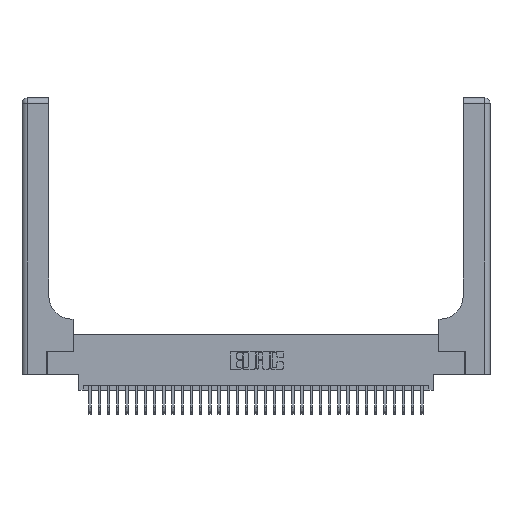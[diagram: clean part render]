
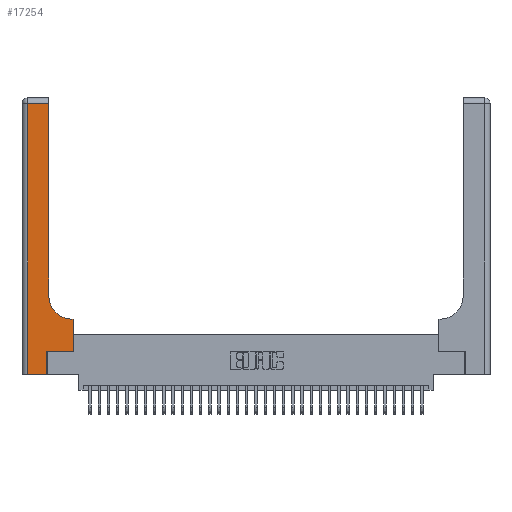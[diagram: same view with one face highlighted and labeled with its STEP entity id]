
A CAD part, top view. The second image highlights one B-rep face of the part: STEP entity #17254.
In plain terms, the highlighted planar face has unit normal (0, 0, 1).
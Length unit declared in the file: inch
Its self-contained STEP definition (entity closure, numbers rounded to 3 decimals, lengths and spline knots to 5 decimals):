
#334 = AXIS2_PLACEMENT_3D ( 'NONE', #34605, #17722, #707 ) ;
#538 = CARTESIAN_POINT ( 'NONE',  ( 0.2915, 0.85, 0.37 ) ) ;
#707 = DIRECTION ( 'NONE',  ( -1., 0., 0. ) ) ;
#1092 = VERTEX_POINT ( 'NONE', #1287 ) ;
#1287 = CARTESIAN_POINT ( 'NONE',  ( 0.269, 0.25, 0.37 ) ) ;
#1878 = EDGE_CURVE ( 'NONE', #11000, #27394, #16429, .T. ) ;
#2353 = EDGE_LOOP ( 'NONE', ( #31193, #34270, #35173, #10606, #19330, #17640, #6904, #22198, #26988 ) ) ;
#4178 = DIRECTION ( 'NONE',  ( 0., 1., 0. ) ) ;
#4311 = EDGE_CURVE ( 'NONE', #13612, #11000, #26911, .T. ) ;
#4938 = LINE ( 'NONE', #35221, #19146 ) ;
#4997 = EDGE_CURVE ( 'NONE', #1092, #9421, #5575, .T. ) ;
#5121 = VERTEX_POINT ( 'NONE', #24001 ) ;
#5575 = LINE ( 'NONE', #29184, #13089 ) ;
#6449 = LINE ( 'NONE', #24709, #34694 ) ;
#6904 = ORIENTED_EDGE ( 'NONE', *, *, #28859, .T. ) ;
#7511 = LINE ( 'NONE', #23362, #35757 ) ;
#8541 = CARTESIAN_POINT ( 'NONE',  ( 0.2915, 2.94, 0.37 ) ) ;
#8618 = EDGE_CURVE ( 'NONE', #27394, #20271, #6449, .T. ) ;
#9202 = PLANE ( 'NONE',  #334 ) ;
#9421 = VERTEX_POINT ( 'NONE', #15098 ) ;
#10004 = AXIS2_PLACEMENT_3D ( 'NONE', #10702, #30483, #13531 ) ;
#10589 = DIRECTION ( 'NONE',  ( 0., 1., 0. ) ) ;
#10606 = ORIENTED_EDGE ( 'NONE', *, *, #31074, .T. ) ;
#10702 = CARTESIAN_POINT ( 'NONE',  ( 0.5415, 0.85, 0.37 ) ) ;
#11000 = VERTEX_POINT ( 'NONE', #36220 ) ;
#12005 = DIRECTION ( 'NONE',  ( -1., 0., 0. ) ) ;
#12429 = CARTESIAN_POINT ( 'NONE',  ( 0.06, 2.94, 0.37 ) ) ;
#13089 = VECTOR ( 'NONE', #15062, 39.37008 ) ;
#13531 = DIRECTION ( 'NONE',  ( 1., 0., 0. ) ) ;
#13612 = VERTEX_POINT ( 'NONE', #30151 ) ;
#13981 = DIRECTION ( 'NONE',  ( -1., 0., 0. ) ) ;
#14082 = VECTOR ( 'NONE', #15932, 39.37008 ) ;
#14226 = FACE_OUTER_BOUND ( 'NONE', #2353, .T. ) ;
#14783 = DIRECTION ( 'NONE',  ( 0., -1., 0. ) ) ;
#14954 = LINE ( 'NONE', #35663, #14082 ) ;
#15062 = DIRECTION ( 'NONE',  ( 1., 0., 0. ) ) ;
#15098 = CARTESIAN_POINT ( 'NONE',  ( 0.5585, 0.25, 0.37 ) ) ;
#15932 = DIRECTION ( 'NONE',  ( 1., 0., 0. ) ) ;
#16429 = CIRCLE ( 'NONE', #10004, 0.25 ) ;
#17254 = ADVANCED_FACE ( 'NONE', ( #14226 ), #9202, .F. ) ;
#17640 = ORIENTED_EDGE ( 'NONE', *, *, #4997, .T. ) ;
#17712 = CARTESIAN_POINT ( 'NONE',  ( 0.2915, 0.6, 0.37 ) ) ;
#17722 = DIRECTION ( 'NONE',  ( 0., 0., -1. ) ) ;
#19146 = VECTOR ( 'NONE', #4178, 39.37008 ) ;
#19330 = ORIENTED_EDGE ( 'NONE', *, *, #27661, .T. ) ;
#20271 = VERTEX_POINT ( 'NONE', #8541 ) ;
#20566 = LINE ( 'NONE', #30052, #21463 ) ;
#21463 = VECTOR ( 'NONE', #32751, 39.37008 ) ;
#22198 = ORIENTED_EDGE ( 'NONE', *, *, #4311, .T. ) ;
#23362 = CARTESIAN_POINT ( 'NONE',  ( 0.06, 3., 0.37 ) ) ;
#24001 = CARTESIAN_POINT ( 'NONE',  ( 0.269, 0., 0.37 ) ) ;
#24709 = CARTESIAN_POINT ( 'NONE',  ( 0.2915, 3., 0.37 ) ) ;
#25024 = CARTESIAN_POINT ( 'NONE',  ( 0., 2.94, 0.37 ) ) ;
#26911 = LINE ( 'NONE', #17712, #33496 ) ;
#26988 = ORIENTED_EDGE ( 'NONE', *, *, #1878, .T. ) ;
#27394 = VERTEX_POINT ( 'NONE', #538 ) ;
#27661 = EDGE_CURVE ( 'NONE', #5121, #1092, #20566, .T. ) ;
#27914 = CARTESIAN_POINT ( 'NONE',  ( 0.06, 0., 0.37 ) ) ;
#27997 = LINE ( 'NONE', #25024, #35433 ) ;
#28859 = EDGE_CURVE ( 'NONE', #9421, #13612, #4938, .T. ) ;
#29081 = EDGE_CURVE ( 'NONE', #20271, #34041, #27997, .T. ) ;
#29184 = CARTESIAN_POINT ( 'NONE',  ( 0.269, 0.25, 0.37 ) ) ;
#30052 = CARTESIAN_POINT ( 'NONE',  ( 0.269, 0., 0.37 ) ) ;
#30151 = CARTESIAN_POINT ( 'NONE',  ( 0.5585, 0.6, 0.37 ) ) ;
#30483 = DIRECTION ( 'NONE',  ( 0., 0., -1. ) ) ;
#31074 = EDGE_CURVE ( 'NONE', #31942, #5121, #14954, .T. ) ;
#31193 = ORIENTED_EDGE ( 'NONE', *, *, #8618, .T. ) ;
#31942 = VERTEX_POINT ( 'NONE', #27914 ) ;
#32751 = DIRECTION ( 'NONE',  ( 0., 1., 0. ) ) ;
#33496 = VECTOR ( 'NONE', #12005, 39.37008 ) ;
#34041 = VERTEX_POINT ( 'NONE', #12429 ) ;
#34270 = ORIENTED_EDGE ( 'NONE', *, *, #29081, .T. ) ;
#34605 = CARTESIAN_POINT ( 'NONE',  ( 0., 3., 0.37 ) ) ;
#34694 = VECTOR ( 'NONE', #10589, 39.37008 ) ;
#35173 = ORIENTED_EDGE ( 'NONE', *, *, #36659, .T. ) ;
#35221 = CARTESIAN_POINT ( 'NONE',  ( 0.5585, 0.25, 0.37 ) ) ;
#35433 = VECTOR ( 'NONE', #13981, 39.37008 ) ;
#35663 = CARTESIAN_POINT ( 'NONE',  ( 0., 0., 0.37 ) ) ;
#35757 = VECTOR ( 'NONE', #14783, 39.37008 ) ;
#36220 = CARTESIAN_POINT ( 'NONE',  ( 0.5415, 0.6, 0.37 ) ) ;
#36659 = EDGE_CURVE ( 'NONE', #34041, #31942, #7511, .T. ) ;
